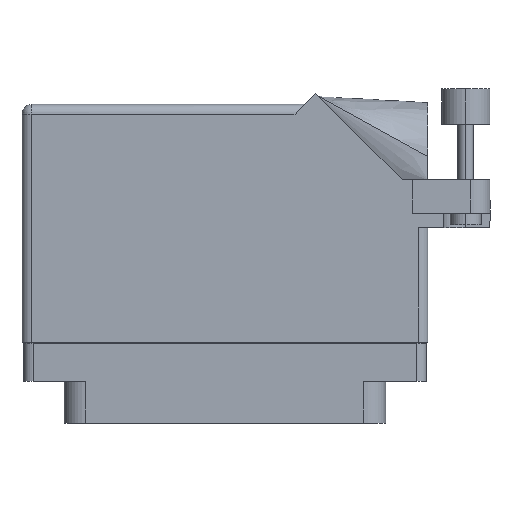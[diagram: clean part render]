
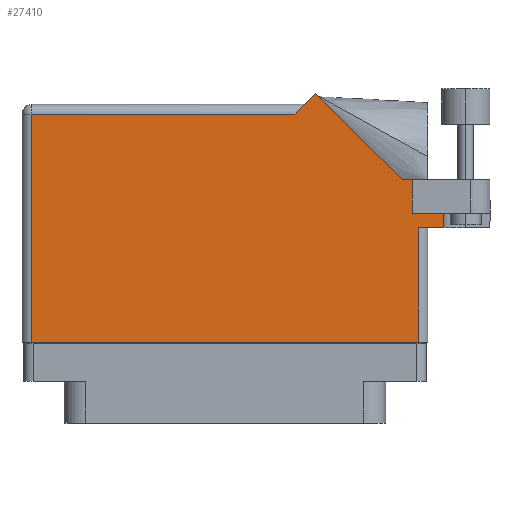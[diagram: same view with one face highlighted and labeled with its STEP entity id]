
A CAD part, front view. The second image highlights one B-rep face of the part: STEP entity #27410.
In plain terms, the highlighted face is planar.
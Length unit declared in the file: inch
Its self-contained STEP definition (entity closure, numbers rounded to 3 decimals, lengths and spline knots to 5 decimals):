
#431 = ORIENTED_EDGE ( 'NONE', *, *, #29322, .T. ) ;
#971 = CARTESIAN_POINT ( 'NONE',  ( 0.58371, 1.50071, 0.455 ) ) ;
#2148 = FACE_OUTER_BOUND ( 'NONE', #38926, .T. ) ;
#2505 = LINE ( 'NONE', #11073, #32193 ) ;
#2943 = VECTOR ( 'NONE', #33810, 39.37008 ) ;
#3009 = LINE ( 'NONE', #42529, #24474 ) ;
#3093 = EDGE_CURVE ( 'NONE', #22512, #7029, #3009, .T. ) ;
#3124 = VECTOR ( 'NONE', #45445, 39.37008 ) ;
#3425 = VECTOR ( 'NONE', #14761, 39.37008 ) ;
#4080 = PLANE ( 'NONE',  #20698 ) ;
#4465 = ORIENTED_EDGE ( 'NONE', *, *, #3093, .T. ) ;
#5485 = DIRECTION ( 'NONE',  ( -0.707, 0.707, 0. ) ) ;
#5549 = ORIENTED_EDGE ( 'NONE', *, *, #20739, .F. ) ;
#5759 = VERTEX_POINT ( 'NONE', #26378 ) ;
#6556 = ORIENTED_EDGE ( 'NONE', *, *, #42247, .T. ) ;
#6652 = LINE ( 'NONE', #32797, #44998 ) ;
#7029 = VERTEX_POINT ( 'NONE', #971 ) ;
#7468 = DIRECTION ( 'NONE',  ( 0., 0., -1. ) ) ;
#7710 = EDGE_CURVE ( 'NONE', #21243, #19000, #6652, .T. ) ;
#7775 = CARTESIAN_POINT ( 'NONE',  ( -1.306, 1.43, 0.455 ) ) ;
#7834 = DIRECTION ( 'NONE',  ( 1., 0., 0. ) ) ;
#8080 = CARTESIAN_POINT ( 'NONE',  ( 1.4075, 1.06177, 0.455 ) ) ;
#8567 = VERTEX_POINT ( 'NONE', #41215 ) ;
#8744 = CARTESIAN_POINT ( 'NONE',  ( 1.244, -0.1, 0.455 ) ) ;
#9967 = EDGE_CURVE ( 'NONE', #18189, #22512, #44722, .T. ) ;
#10361 = LINE ( 'NONE', #38102, #24319 ) ;
#10842 = CARTESIAN_POINT ( 'NONE',  ( -1.244, -0.1, 0.455 ) ) ;
#11073 = CARTESIAN_POINT ( 'NONE',  ( 1.206, 0.731, 0.455 ) ) ;
#11101 = EDGE_CURVE ( 'NONE', #5759, #21243, #28982, .T. ) ;
#12182 = VERTEX_POINT ( 'NONE', #22383 ) ;
#12425 = ORIENTED_EDGE ( 'NONE', *, *, #32537, .T. ) ;
#12779 = VERTEX_POINT ( 'NONE', #18391 ) ;
#13017 = CARTESIAN_POINT ( 'NONE',  ( 1.244, 0.637, 0.455 ) ) ;
#14266 = DIRECTION ( 'NONE',  ( 1., 0., 0. ) ) ;
#14420 = ORIENTED_EDGE ( 'NONE', *, *, #9967, .T. ) ;
#14761 = DIRECTION ( 'NONE',  ( 0., -1., 0. ) ) ;
#15088 = EDGE_CURVE ( 'NONE', #12779, #8567, #39610, .T. ) ;
#15281 = VECTOR ( 'NONE', #24226, 39.37008 ) ;
#17357 = LINE ( 'NONE', #39354, #45305 ) ;
#17393 = VECTOR ( 'NONE', #28779, 39.37008 ) ;
#17811 = EDGE_CURVE ( 'NONE', #18747, #18189, #10361, .T. ) ;
#18189 = VERTEX_POINT ( 'NONE', #34874 ) ;
#18391 = CARTESIAN_POINT ( 'NONE',  ( 1.4075, 0.731, 0.455 ) ) ;
#18747 = VERTEX_POINT ( 'NONE', #20898 ) ;
#19000 = VERTEX_POINT ( 'NONE', #8744 ) ;
#19412 = CARTESIAN_POINT ( 'NONE',  ( -1.306, 1.368, 0.455 ) ) ;
#19682 = ORIENTED_EDGE ( 'NONE', *, *, #15088, .F. ) ;
#19954 = ORIENTED_EDGE ( 'NONE', *, *, #36160, .T. ) ;
#20698 = AXIS2_PLACEMENT_3D ( 'NONE', #7775, #7468, #22436 ) ;
#20739 = EDGE_CURVE ( 'NONE', #18747, #12779, #2505, .T. ) ;
#20898 = CARTESIAN_POINT ( 'NONE',  ( 1.206, 0.731, 0.455 ) ) ;
#21190 = ORIENTED_EDGE ( 'NONE', *, *, #7710, .T. ) ;
#21243 = VERTEX_POINT ( 'NONE', #38624 ) ;
#22383 = CARTESIAN_POINT ( 'NONE',  ( 0.451, 1.368, 0.455 ) ) ;
#22436 = DIRECTION ( 'NONE',  ( -1., 0., 0. ) ) ;
#22512 = VERTEX_POINT ( 'NONE', #46202 ) ;
#24226 = DIRECTION ( 'NONE',  ( 0., 1., 0. ) ) ;
#24319 = VECTOR ( 'NONE', #38580, 39.37008 ) ;
#24474 = VECTOR ( 'NONE', #5485, 39.37008 ) ;
#25155 = LINE ( 'NONE', #13017, #15281 ) ;
#26378 = CARTESIAN_POINT ( 'NONE',  ( -1.244, 1.368, 0.455 ) ) ;
#27410 = ADVANCED_FACE ( 'NONE', ( #2148 ), #4080, .F. ) ;
#27949 = CARTESIAN_POINT ( 'NONE',  ( 1.244, 0.637, 0.455 ) ) ;
#28779 = DIRECTION ( 'NONE',  ( -1., 0., 0. ) ) ;
#28982 = LINE ( 'NONE', #10842, #3425 ) ;
#29322 = EDGE_CURVE ( 'NONE', #12182, #5759, #45228, .T. ) ;
#29863 = LINE ( 'NONE', #37657, #3124 ) ;
#31165 = ORIENTED_EDGE ( 'NONE', *, *, #17811, .T. ) ;
#32193 = VECTOR ( 'NONE', #7834, 39.37008 ) ;
#32537 = EDGE_CURVE ( 'NONE', #19000, #32612, #25155, .T. ) ;
#32612 = VERTEX_POINT ( 'NONE', #27949 ) ;
#32797 = CARTESIAN_POINT ( 'NONE',  ( -1.306, -0.1, 0.455 ) ) ;
#33810 = DIRECTION ( 'NONE',  ( 0., -1., 0. ) ) ;
#34874 = CARTESIAN_POINT ( 'NONE',  ( 1.206, 0.944, 0.455 ) ) ;
#36160 = EDGE_CURVE ( 'NONE', #32612, #8567, #29863, .T. ) ;
#37657 = CARTESIAN_POINT ( 'NONE',  ( 1.306, 0.637, 0.455 ) ) ;
#38102 = CARTESIAN_POINT ( 'NONE',  ( 1.206, 0.731, 0.455 ) ) ;
#38104 = DIRECTION ( 'NONE',  ( -1., 0., 0. ) ) ;
#38580 = DIRECTION ( 'NONE',  ( 0., 1., 0. ) ) ;
#38624 = CARTESIAN_POINT ( 'NONE',  ( -1.244, -0.1, 0.455 ) ) ;
#38926 = EDGE_LOOP ( 'NONE', ( #21190, #12425, #19954, #19682, #5549, #31165, #14420, #4465, #6556, #431, #45182 ) ) ;
#39354 = CARTESIAN_POINT ( 'NONE',  ( 0.513, 1.43, 0.455 ) ) ;
#39610 = LINE ( 'NONE', #8080, #2943 ) ;
#39868 = CARTESIAN_POINT ( 'NONE',  ( 1.706, 0.944, 0.455 ) ) ;
#40572 = VECTOR ( 'NONE', #38104, 39.37008 ) ;
#41215 = CARTESIAN_POINT ( 'NONE',  ( 1.4075, 0.637, 0.455 ) ) ;
#42247 = EDGE_CURVE ( 'NONE', #7029, #12182, #17357, .T. ) ;
#42529 = CARTESIAN_POINT ( 'NONE',  ( 1.14042, 0.944, 0.455 ) ) ;
#42778 = DIRECTION ( 'NONE',  ( -0.707, -0.707, 0. ) ) ;
#44722 = LINE ( 'NONE', #39868, #17393 ) ;
#44998 = VECTOR ( 'NONE', #14266, 39.37008 ) ;
#45182 = ORIENTED_EDGE ( 'NONE', *, *, #11101, .T. ) ;
#45228 = LINE ( 'NONE', #19412, #40572 ) ;
#45305 = VECTOR ( 'NONE', #42778, 39.37008 ) ;
#45445 = DIRECTION ( 'NONE',  ( 1., 0., 0. ) ) ;
#46202 = CARTESIAN_POINT ( 'NONE',  ( 1.14042, 0.944, 0.455 ) ) ;
